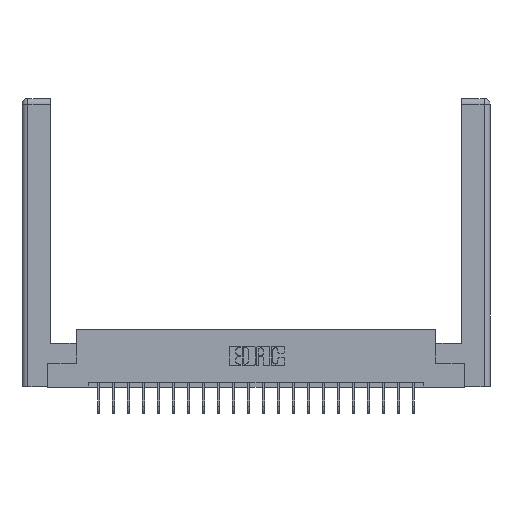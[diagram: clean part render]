
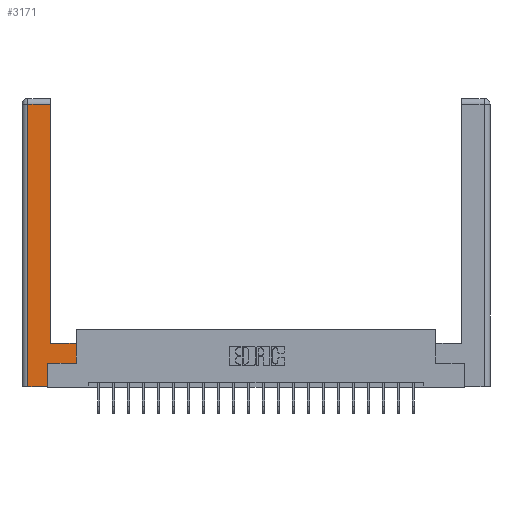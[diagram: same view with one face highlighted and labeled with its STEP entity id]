
A CAD part, top view. The second image highlights one B-rep face of the part: STEP entity #3171.
In plain terms, the highlighted planar face has unit normal (0, 0, 1).
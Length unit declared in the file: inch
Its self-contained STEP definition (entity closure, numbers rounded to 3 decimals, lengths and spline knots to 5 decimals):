
#462 = CARTESIAN_POINT ( 'NONE',  ( 0.265, 0.245, 0. ) ) ;
#1358 = DIRECTION ( 'NONE',  ( 1., 0., 0. ) ) ;
#1663 = VECTOR ( 'NONE', #18055, 39.37008 ) ;
#2410 = DIRECTION ( 'NONE',  ( -1., 0., 0. ) ) ;
#2579 = VERTEX_POINT ( 'NONE', #17952 ) ;
#2655 = VERTEX_POINT ( 'NONE', #9231 ) ;
#2665 = ORIENTED_EDGE ( 'NONE', *, *, #23387, .T. ) ;
#2853 = LINE ( 'NONE', #10867, #1663 ) ;
#3020 = DIRECTION ( 'NONE',  ( 0., 0., -1. ) ) ;
#3171 = ADVANCED_FACE ( 'NONE', ( #22772 ), #21001, .F. ) ;
#3544 = CARTESIAN_POINT ( 'NONE',  ( 0.265, 0.245, 0. ) ) ;
#5137 = EDGE_LOOP ( 'NONE', ( #9539, #7346, #9302, #2665, #11983, #19171, #12882, #15887 ) ) ;
#5244 = DIRECTION ( 'NONE',  ( 0., -1., 0. ) ) ;
#5944 = LINE ( 'NONE', #3544, #17509 ) ;
#6108 = VERTEX_POINT ( 'NONE', #7870 ) ;
#6738 = DIRECTION ( 'NONE',  ( -1., 0., 0. ) ) ;
#6789 = CARTESIAN_POINT ( 'NONE',  ( 0.0615, 0., 0. ) ) ;
#7346 = ORIENTED_EDGE ( 'NONE', *, *, #10387, .T. ) ;
#7377 = VERTEX_POINT ( 'NONE', #9680 ) ;
#7870 = CARTESIAN_POINT ( 'NONE',  ( 0.0615, 2.94, 0. ) ) ;
#8189 = VECTOR ( 'NONE', #1358, 39.37008 ) ;
#8384 = LINE ( 'NONE', #16390, #13622 ) ;
#9231 = CARTESIAN_POINT ( 'NONE',  ( 0.565, 0.245, 0. ) ) ;
#9302 = ORIENTED_EDGE ( 'NONE', *, *, #20467, .T. ) ;
#9539 = ORIENTED_EDGE ( 'NONE', *, *, #10160, .T. ) ;
#9598 = CARTESIAN_POINT ( 'NONE',  ( 0.265, 0., 0. ) ) ;
#9680 = CARTESIAN_POINT ( 'NONE',  ( 0.295, 2.94, 0. ) ) ;
#10160 = EDGE_CURVE ( 'NONE', #10923, #7377, #8384, .T. ) ;
#10387 = EDGE_CURVE ( 'NONE', #7377, #6108, #14460, .T. ) ;
#10638 = LINE ( 'NONE', #21853, #14676 ) ;
#10867 = CARTESIAN_POINT ( 'NONE',  ( 0.565, 0.45, 0. ) ) ;
#10886 = VERTEX_POINT ( 'NONE', #462 ) ;
#10923 = VERTEX_POINT ( 'NONE', #12311 ) ;
#11625 = EDGE_CURVE ( 'NONE', #2579, #10923, #23703, .T. ) ;
#11983 = ORIENTED_EDGE ( 'NONE', *, *, #15793, .T. ) ;
#12250 = CARTESIAN_POINT ( 'NONE',  ( 0.0615, 2.94, 0. ) ) ;
#12311 = CARTESIAN_POINT ( 'NONE',  ( 0.295, 0.45, 0. ) ) ;
#12489 = CARTESIAN_POINT ( 'NONE',  ( 0.565, 0.245, 0. ) ) ;
#12882 = ORIENTED_EDGE ( 'NONE', *, *, #22376, .T. ) ;
#13027 = VERTEX_POINT ( 'NONE', #6789 ) ;
#13622 = VECTOR ( 'NONE', #23650, 39.37008 ) ;
#13699 = LINE ( 'NONE', #12489, #8189 ) ;
#14105 = LINE ( 'NONE', #22339, #21980 ) ;
#14460 = LINE ( 'NONE', #12250, #21434 ) ;
#14676 = VECTOR ( 'NONE', #5244, 39.37008 ) ;
#14926 = DIRECTION ( 'NONE',  ( 1., 0., 0. ) ) ;
#15793 = EDGE_CURVE ( 'NONE', #15927, #10886, #5944, .T. ) ;
#15887 = ORIENTED_EDGE ( 'NONE', *, *, #11625, .T. ) ;
#15927 = VERTEX_POINT ( 'NONE', #9598 ) ;
#15984 = DIRECTION ( 'NONE',  ( -1., 0., 0. ) ) ;
#16390 = CARTESIAN_POINT ( 'NONE',  ( 0.295, 3., 0. ) ) ;
#17049 = EDGE_CURVE ( 'NONE', #10886, #2655, #13699, .T. ) ;
#17509 = VECTOR ( 'NONE', #23781, 39.37008 ) ;
#17952 = CARTESIAN_POINT ( 'NONE',  ( 0.565, 0.45, 0. ) ) ;
#18055 = DIRECTION ( 'NONE',  ( 0., 1., 0. ) ) ;
#19171 = ORIENTED_EDGE ( 'NONE', *, *, #17049, .T. ) ;
#19650 = CARTESIAN_POINT ( 'NONE',  ( 0., 0., 0. ) ) ;
#20134 = AXIS2_PLACEMENT_3D ( 'NONE', #19650, #3020, #15984 ) ;
#20467 = EDGE_CURVE ( 'NONE', #6108, #13027, #10638, .T. ) ;
#20832 = CARTESIAN_POINT ( 'NONE',  ( 0.295, 0.45, 0. ) ) ;
#21001 = PLANE ( 'NONE',  #20134 ) ;
#21363 = VECTOR ( 'NONE', #2410, 39.37008 ) ;
#21434 = VECTOR ( 'NONE', #6738, 39.37008 ) ;
#21853 = CARTESIAN_POINT ( 'NONE',  ( 0.0615, 0., 0. ) ) ;
#21980 = VECTOR ( 'NONE', #14926, 39.37008 ) ;
#22339 = CARTESIAN_POINT ( 'NONE',  ( 0.265, 0., 0. ) ) ;
#22376 = EDGE_CURVE ( 'NONE', #2655, #2579, #2853, .T. ) ;
#22772 = FACE_OUTER_BOUND ( 'NONE', #5137, .T. ) ;
#23387 = EDGE_CURVE ( 'NONE', #13027, #15927, #14105, .T. ) ;
#23650 = DIRECTION ( 'NONE',  ( 0., 1., 0. ) ) ;
#23703 = LINE ( 'NONE', #20832, #21363 ) ;
#23781 = DIRECTION ( 'NONE',  ( 0., 1., 0. ) ) ;
